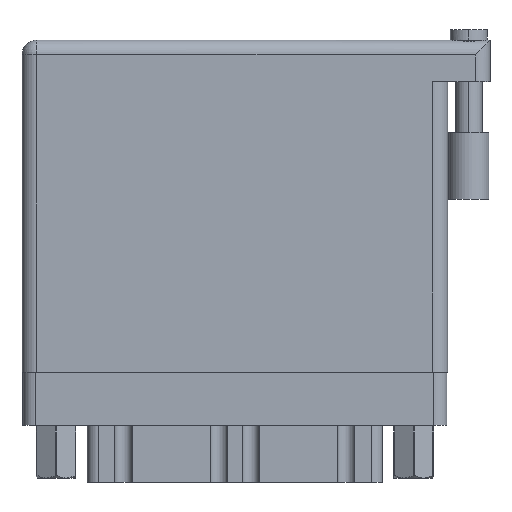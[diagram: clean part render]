
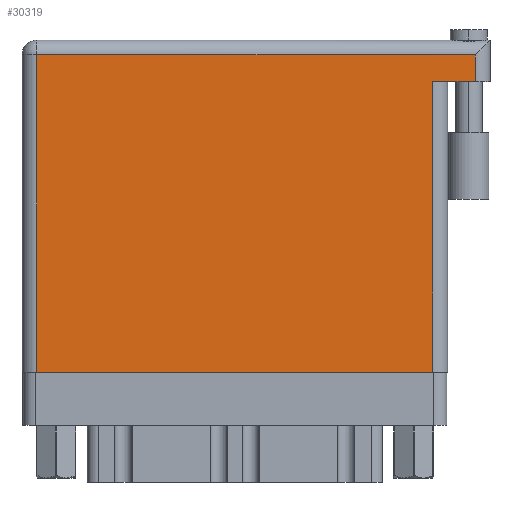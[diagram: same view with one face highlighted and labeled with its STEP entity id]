
A CAD part, front view. The second image highlights one B-rep face of the part: STEP entity #30319.
In plain terms, the highlighted face is planar.
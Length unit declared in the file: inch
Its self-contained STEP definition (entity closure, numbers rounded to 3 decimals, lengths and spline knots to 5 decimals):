
#568 = DIRECTION ( 'NONE',  ( 0., 1., 0. ) ) ;
#632 = CARTESIAN_POINT ( 'NONE',  ( 2.208, 1.369, 0. ) ) ;
#2848 = LINE ( 'NONE', #13632, #3951 ) ;
#3005 = CARTESIAN_POINT ( 'NONE',  ( 0.07, 1.496, 0. ) ) ;
#3766 = EDGE_CURVE ( 'NONE', #12105, #22919, #5937, .T. ) ;
#3951 = VECTOR ( 'NONE', #46614, 39.37008 ) ;
#4282 = DIRECTION ( 'NONE',  ( 0., 1., 0. ) ) ;
#4782 = PLANE ( 'NONE',  #26240 ) ;
#5050 = ORIENTED_EDGE ( 'NONE', *, *, #9940, .F. ) ;
#5169 = CARTESIAN_POINT ( 'NONE',  ( 2.138, 1.496, 0. ) ) ;
#5463 = VERTEX_POINT ( 'NONE', #45783 ) ;
#5937 = LINE ( 'NONE', #31334, #38116 ) ;
#6015 = LINE ( 'NONE', #13442, #11235 ) ;
#6292 = VECTOR ( 'NONE', #41051, 39.37008 ) ;
#6582 = EDGE_CURVE ( 'NONE', #27363, #12105, #21892, .T. ) ;
#6803 = EDGE_LOOP ( 'NONE', ( #21356, #25436, #5050, #42727, #42777, #7576 ) ) ;
#7576 = ORIENTED_EDGE ( 'NONE', *, *, #46620, .T. ) ;
#9940 = EDGE_CURVE ( 'NONE', #27363, #5463, #45100, .T. ) ;
#10551 = DIRECTION ( 'NONE',  ( 0., -1., 0. ) ) ;
#11081 = CARTESIAN_POINT ( 'NONE',  ( 2.138, 1.566, 0. ) ) ;
#11235 = VECTOR ( 'NONE', #10551, 39.37008 ) ;
#12105 = VERTEX_POINT ( 'NONE', #5169 ) ;
#13442 = CARTESIAN_POINT ( 'NONE',  ( 0.07, 0., 0. ) ) ;
#13632 = CARTESIAN_POINT ( 'NONE',  ( 0., 0., 0. ) ) ;
#14353 = EDGE_CURVE ( 'NONE', #45855, #5463, #32095, .T. ) ;
#15820 = FACE_OUTER_BOUND ( 'NONE', #6803, .T. ) ;
#16051 = CARTESIAN_POINT ( 'NONE',  ( 0., 1.566, 0. ) ) ;
#18814 = CARTESIAN_POINT ( 'NONE',  ( 1.938, 0., 0. ) ) ;
#19413 = DIRECTION ( 'NONE',  ( -1., 0., 0. ) ) ;
#21356 = ORIENTED_EDGE ( 'NONE', *, *, #38520, .T. ) ;
#21892 = LINE ( 'NONE', #11081, #32317 ) ;
#22829 = CARTESIAN_POINT ( 'NONE',  ( 2.138, 1.369, 0. ) ) ;
#22919 = VERTEX_POINT ( 'NONE', #3005 ) ;
#23039 = VERTEX_POINT ( 'NONE', #33634 ) ;
#23489 = DIRECTION ( 'NONE',  ( 0., 0., -1. ) ) ;
#25436 = ORIENTED_EDGE ( 'NONE', *, *, #14353, .T. ) ;
#26240 = AXIS2_PLACEMENT_3D ( 'NONE', #16051, #23489, #19413 ) ;
#26397 = VECTOR ( 'NONE', #4282, 39.37008 ) ;
#27363 = VERTEX_POINT ( 'NONE', #22829 ) ;
#28521 = CARTESIAN_POINT ( 'NONE',  ( 1.938, 1.369, 0. ) ) ;
#30319 = ADVANCED_FACE ( 'NONE', ( #15820 ), #4782, .F. ) ;
#31334 = CARTESIAN_POINT ( 'NONE',  ( 0., 1.496, 0. ) ) ;
#32095 = LINE ( 'NONE', #28521, #26397 ) ;
#32317 = VECTOR ( 'NONE', #568, 39.37008 ) ;
#33634 = CARTESIAN_POINT ( 'NONE',  ( 0.07, 0., 0. ) ) ;
#38116 = VECTOR ( 'NONE', #41347, 39.37008 ) ;
#38520 = EDGE_CURVE ( 'NONE', #23039, #45855, #2848, .T. ) ;
#41051 = DIRECTION ( 'NONE',  ( -1., 0., 0. ) ) ;
#41347 = DIRECTION ( 'NONE',  ( -1., 0., 0. ) ) ;
#42727 = ORIENTED_EDGE ( 'NONE', *, *, #6582, .T. ) ;
#42777 = ORIENTED_EDGE ( 'NONE', *, *, #3766, .T. ) ;
#45100 = LINE ( 'NONE', #632, #6292 ) ;
#45783 = CARTESIAN_POINT ( 'NONE',  ( 1.938, 1.369, 0. ) ) ;
#45855 = VERTEX_POINT ( 'NONE', #18814 ) ;
#46614 = DIRECTION ( 'NONE',  ( 1., 0., 0. ) ) ;
#46620 = EDGE_CURVE ( 'NONE', #22919, #23039, #6015, .T. ) ;
